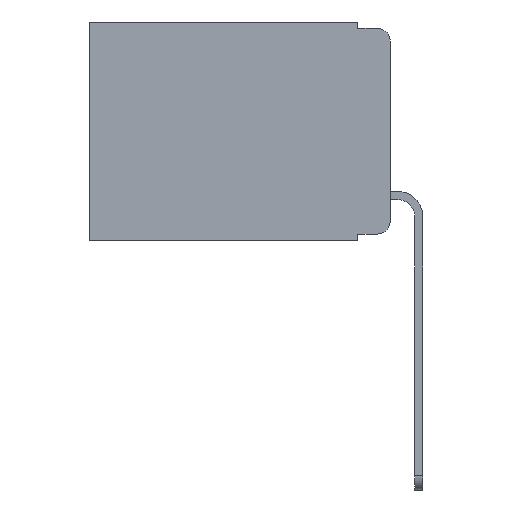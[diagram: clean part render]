
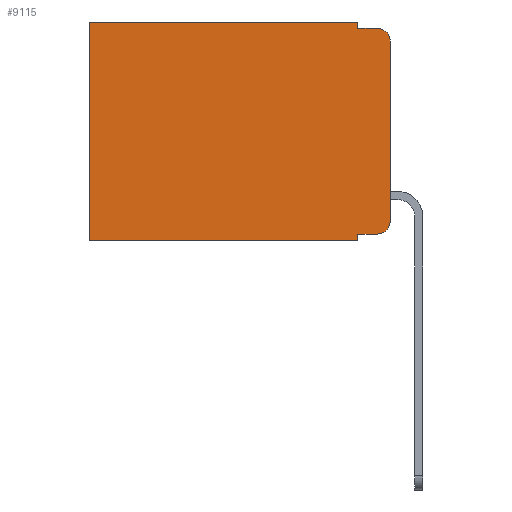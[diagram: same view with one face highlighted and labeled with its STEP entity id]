
A CAD part, left-side view. The second image highlights one B-rep face of the part: STEP entity #9115.
In plain terms, the highlighted planar face has unit normal (-1, 0, 0).
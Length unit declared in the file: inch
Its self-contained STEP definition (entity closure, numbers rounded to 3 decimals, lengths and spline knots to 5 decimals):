
#272 = LINE ( 'NONE', #11795, #3292 ) ;
#697 = DIRECTION ( 'NONE',  ( 0., 1., 0. ) ) ;
#700 = ORIENTED_EDGE ( 'NONE', *, *, #2893, .T. ) ;
#886 = CARTESIAN_POINT ( 'NONE',  ( 0.298, 0.02, -0.01 ) ) ;
#1114 = FACE_OUTER_BOUND ( 'NONE', #6309, .T. ) ;
#1217 = EDGE_CURVE ( 'NONE', #9488, #3482, #4068, .T. ) ;
#1468 = EDGE_CURVE ( 'NONE', #1475, #7939, #272, .T. ) ;
#1475 = VERTEX_POINT ( 'NONE', #11876 ) ;
#1517 = VECTOR ( 'NONE', #1683, 39.37008 ) ;
#1552 = CARTESIAN_POINT ( 'NONE',  ( 0.298, 0.473, 0. ) ) ;
#1574 = ORIENTED_EDGE ( 'NONE', *, *, #11526, .T. ) ;
#1683 = DIRECTION ( 'NONE',  ( 0., -1., 0. ) ) ;
#1754 = ORIENTED_EDGE ( 'NONE', *, *, #10290, .T. ) ;
#1823 = CARTESIAN_POINT ( 'NONE',  ( 0.298, 0.051, -0.343 ) ) ;
#1842 = DIRECTION ( 'NONE',  ( -1., 0., 0. ) ) ;
#1860 = LINE ( 'NONE', #2968, #7084 ) ;
#2004 = ORIENTED_EDGE ( 'NONE', *, *, #9664, .F. ) ;
#2384 = ORIENTED_EDGE ( 'NONE', *, *, #2496, .T. ) ;
#2406 = LINE ( 'NONE', #6126, #7284 ) ;
#2422 = PLANE ( 'NONE',  #3507 ) ;
#2496 = EDGE_CURVE ( 'NONE', #5684, #11001, #9512, .T. ) ;
#2893 = EDGE_CURVE ( 'NONE', #8362, #5684, #1860, .T. ) ;
#2968 = CARTESIAN_POINT ( 'NONE',  ( 0.298, 0., 0. ) ) ;
#3292 = VECTOR ( 'NONE', #11949, 39.37008 ) ;
#3326 = VERTEX_POINT ( 'NONE', #4079 ) ;
#3387 = CARTESIAN_POINT ( 'NONE',  ( 0.298, 0., 0. ) ) ;
#3482 = VERTEX_POINT ( 'NONE', #10011 ) ;
#3507 = AXIS2_PLACEMENT_3D ( 'NONE', #3387, #10023, #4379 ) ;
#3523 = CARTESIAN_POINT ( 'NONE',  ( 0.298, 0., -0.03 ) ) ;
#4068 = LINE ( 'NONE', #5594, #9109 ) ;
#4079 = CARTESIAN_POINT ( 'NONE',  ( 0.298, 0.02, -0.333 ) ) ;
#4165 = LINE ( 'NONE', #10238, #1517 ) ;
#4209 = VECTOR ( 'NONE', #6719, 39.37008 ) ;
#4314 = ORIENTED_EDGE ( 'NONE', *, *, #1217, .F. ) ;
#4379 = DIRECTION ( 'NONE',  ( 0., 0., -1. ) ) ;
#4521 = LINE ( 'NONE', #9479, #4209 ) ;
#4724 = VERTEX_POINT ( 'NONE', #886 ) ;
#5161 = EDGE_CURVE ( 'NONE', #7939, #11001, #10718, .T. ) ;
#5326 = EDGE_CURVE ( 'NONE', #9488, #4724, #9273, .T. ) ;
#5525 = EDGE_CURVE ( 'NONE', #8452, #4724, #2406, .T. ) ;
#5594 = CARTESIAN_POINT ( 'NONE',  ( 0.298, 0., 0. ) ) ;
#5684 = VERTEX_POINT ( 'NONE', #7973 ) ;
#5768 = CARTESIAN_POINT ( 'NONE',  ( 0.298, 0.473, -0.343 ) ) ;
#5894 = CARTESIAN_POINT ( 'NONE',  ( 0.298, 0.02, -0.03 ) ) ;
#6126 = CARTESIAN_POINT ( 'NONE',  ( 0.298, 0.051, -0.01 ) ) ;
#6309 = EDGE_LOOP ( 'NONE', ( #4314, #10969, #11461, #2004, #700, #2384, #7608, #12048, #1574, #1754 ) ) ;
#6340 = DIRECTION ( 'NONE',  ( 0., 0., -1. ) ) ;
#6719 = DIRECTION ( 'NONE',  ( 0., 0., -1. ) ) ;
#6911 = DIRECTION ( 'NONE',  ( 0., 0., -1. ) ) ;
#7084 = VECTOR ( 'NONE', #8757, 39.37008 ) ;
#7284 = VECTOR ( 'NONE', #8020, 39.37008 ) ;
#7608 = ORIENTED_EDGE ( 'NONE', *, *, #5161, .F. ) ;
#7669 = CARTESIAN_POINT ( 'NONE',  ( 0.298, 0.02, -0.313 ) ) ;
#7939 = VERTEX_POINT ( 'NONE', #1823 ) ;
#7973 = CARTESIAN_POINT ( 'NONE',  ( 0.298, 0.473, 0. ) ) ;
#8020 = DIRECTION ( 'NONE',  ( 0., -1., 0. ) ) ;
#8282 = VECTOR ( 'NONE', #697, 39.37008 ) ;
#8362 = VERTEX_POINT ( 'NONE', #10868 ) ;
#8452 = VERTEX_POINT ( 'NONE', #10948 ) ;
#8586 = DIRECTION ( 'NONE',  ( 0., 0., -1. ) ) ;
#8757 = DIRECTION ( 'NONE',  ( 0., 1., 0. ) ) ;
#9109 = VECTOR ( 'NONE', #10674, 39.37008 ) ;
#9115 = ADVANCED_FACE ( 'NONE', ( #1114 ), #2422, .F. ) ;
#9273 = CIRCLE ( 'NONE', #10401, 0.02 ) ;
#9382 = CIRCLE ( 'NONE', #10195, 0.02 ) ;
#9479 = CARTESIAN_POINT ( 'NONE',  ( 0.298, 0.051, 0. ) ) ;
#9488 = VERTEX_POINT ( 'NONE', #3523 ) ;
#9512 = LINE ( 'NONE', #1552, #11885 ) ;
#9664 = EDGE_CURVE ( 'NONE', #8362, #8452, #4521, .T. ) ;
#10011 = CARTESIAN_POINT ( 'NONE',  ( 0.298, 0., -0.313 ) ) ;
#10023 = DIRECTION ( 'NONE',  ( 1., 0., 0. ) ) ;
#10195 = AXIS2_PLACEMENT_3D ( 'NONE', #7669, #1842, #8586 ) ;
#10238 = CARTESIAN_POINT ( 'NONE',  ( 0.298, 0.051, -0.333 ) ) ;
#10286 = CARTESIAN_POINT ( 'NONE',  ( 0.298, 0., -0.343 ) ) ;
#10290 = EDGE_CURVE ( 'NONE', #3326, #3482, #9382, .T. ) ;
#10401 = AXIS2_PLACEMENT_3D ( 'NONE', #5894, #12304, #6911 ) ;
#10674 = DIRECTION ( 'NONE',  ( 0., 0., -1. ) ) ;
#10718 = LINE ( 'NONE', #10286, #8282 ) ;
#10868 = CARTESIAN_POINT ( 'NONE',  ( 0.298, 0.051, 0. ) ) ;
#10948 = CARTESIAN_POINT ( 'NONE',  ( 0.298, 0.051, -0.01 ) ) ;
#10969 = ORIENTED_EDGE ( 'NONE', *, *, #5326, .T. ) ;
#11001 = VERTEX_POINT ( 'NONE', #5768 ) ;
#11461 = ORIENTED_EDGE ( 'NONE', *, *, #5525, .F. ) ;
#11526 = EDGE_CURVE ( 'NONE', #1475, #3326, #4165, .T. ) ;
#11795 = CARTESIAN_POINT ( 'NONE',  ( 0.298, 0.051, 0. ) ) ;
#11876 = CARTESIAN_POINT ( 'NONE',  ( 0.298, 0.051, -0.333 ) ) ;
#11885 = VECTOR ( 'NONE', #6340, 39.37008 ) ;
#11949 = DIRECTION ( 'NONE',  ( 0., 0., -1. ) ) ;
#12048 = ORIENTED_EDGE ( 'NONE', *, *, #1468, .F. ) ;
#12304 = DIRECTION ( 'NONE',  ( -1., 0., 0. ) ) ;
